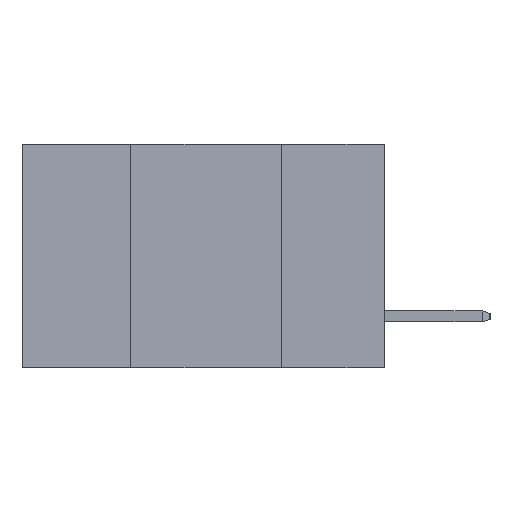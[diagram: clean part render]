
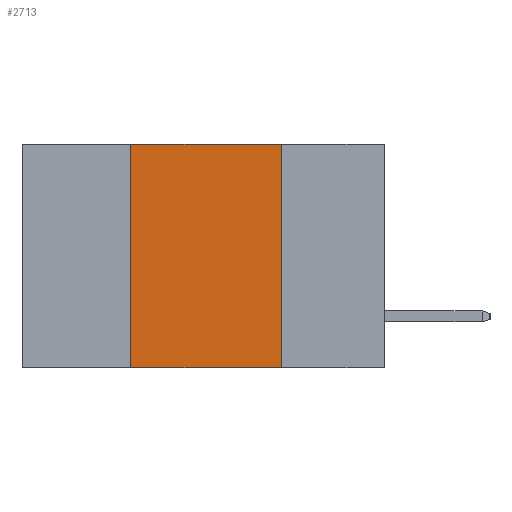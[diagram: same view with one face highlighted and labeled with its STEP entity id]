
A CAD part, left-side view. The second image highlights one B-rep face of the part: STEP entity #2713.
In plain terms, the highlighted planar face has unit normal (-1, 0, 0).
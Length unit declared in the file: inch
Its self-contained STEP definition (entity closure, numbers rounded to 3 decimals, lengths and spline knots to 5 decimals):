
#540 = DIRECTION ( 'NONE',  ( 0., 0., 1. ) ) ;
#859 = CARTESIAN_POINT ( 'NONE',  ( 0., 0.6, 0. ) ) ;
#2713 = ADVANCED_FACE ( 'NONE', ( #28898 ), #15711, .F. ) ;
#3310 = EDGE_LOOP ( 'NONE', ( #9516, #16876, #29978, #12645 ) ) ;
#3330 = DIRECTION ( 'NONE',  ( 1., 0., 0. ) ) ;
#3741 = LINE ( 'NONE', #4847, #16190 ) ;
#3779 = VERTEX_POINT ( 'NONE', #7841 ) ;
#4847 = CARTESIAN_POINT ( 'NONE',  ( 0., 0.6, 0. ) ) ;
#6295 = DIRECTION ( 'NONE',  ( 0., 0., -1. ) ) ;
#6432 = LINE ( 'NONE', #26249, #12292 ) ;
#7841 = CARTESIAN_POINT ( 'NONE',  ( 0., 0.17, 0. ) ) ;
#8009 = CARTESIAN_POINT ( 'NONE',  ( 0., 0.42, 0. ) ) ;
#9329 = CARTESIAN_POINT ( 'NONE',  ( 0., 0.42, 0. ) ) ;
#9516 = ORIENTED_EDGE ( 'NONE', *, *, #13468, .F. ) ;
#11092 = CARTESIAN_POINT ( 'NONE',  ( 0., 0.6, -0.37 ) ) ;
#11458 = EDGE_CURVE ( 'NONE', #31748, #11876, #11743, .T. ) ;
#11743 = LINE ( 'NONE', #11092, #23347 ) ;
#11876 = VERTEX_POINT ( 'NONE', #20063 ) ;
#12292 = VECTOR ( 'NONE', #6295, 39.37008 ) ;
#12645 = ORIENTED_EDGE ( 'NONE', *, *, #11458, .T. ) ;
#13468 = EDGE_CURVE ( 'NONE', #3779, #11876, #6432, .T. ) ;
#13597 = DIRECTION ( 'NONE',  ( 0., -1., 0. ) ) ;
#15711 = PLANE ( 'NONE',  #18337 ) ;
#16190 = VECTOR ( 'NONE', #24708, 39.37008 ) ;
#16876 = ORIENTED_EDGE ( 'NONE', *, *, #18781, .F. ) ;
#18337 = AXIS2_PLACEMENT_3D ( 'NONE', #859, #3330, #20730 ) ;
#18634 = VERTEX_POINT ( 'NONE', #9329 ) ;
#18728 = VECTOR ( 'NONE', #540, 39.37008 ) ;
#18781 = EDGE_CURVE ( 'NONE', #18634, #3779, #3741, .T. ) ;
#18889 = CARTESIAN_POINT ( 'NONE',  ( 0., 0.42, -0.37 ) ) ;
#20063 = CARTESIAN_POINT ( 'NONE',  ( 0., 0.17, -0.37 ) ) ;
#20730 = DIRECTION ( 'NONE',  ( 0., 0., -1. ) ) ;
#23347 = VECTOR ( 'NONE', #13597, 39.37008 ) ;
#24708 = DIRECTION ( 'NONE',  ( 0., -1., 0. ) ) ;
#26249 = CARTESIAN_POINT ( 'NONE',  ( 0., 0.17, 0. ) ) ;
#26907 = LINE ( 'NONE', #8009, #18728 ) ;
#28416 = EDGE_CURVE ( 'NONE', #31748, #18634, #26907, .T. ) ;
#28898 = FACE_OUTER_BOUND ( 'NONE', #3310, .T. ) ;
#29978 = ORIENTED_EDGE ( 'NONE', *, *, #28416, .F. ) ;
#31748 = VERTEX_POINT ( 'NONE', #18889 ) ;
